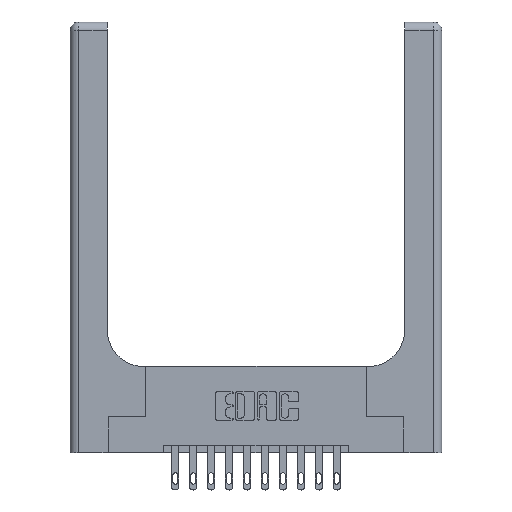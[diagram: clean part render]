
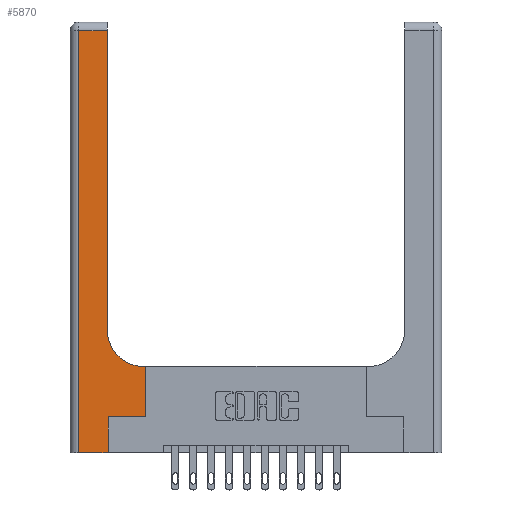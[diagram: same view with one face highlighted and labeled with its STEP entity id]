
A CAD part, top view. The second image highlights one B-rep face of the part: STEP entity #5870.
In plain terms, the highlighted planar face has unit normal (0, 0, 1).
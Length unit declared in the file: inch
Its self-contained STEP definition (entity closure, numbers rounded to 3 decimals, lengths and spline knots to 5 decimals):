
#575 = DIRECTION ( 'NONE',  ( 1., 0., 0. ) ) ;
#804 = LINE ( 'NONE', #5848, #12425 ) ;
#843 = VERTEX_POINT ( 'NONE', #5505 ) ;
#892 = LINE ( 'NONE', #11012, #16225 ) ;
#935 = CARTESIAN_POINT ( 'NONE',  ( 0.51, 0.85, 0.37 ) ) ;
#1201 = ORIENTED_EDGE ( 'NONE', *, *, #14154, .T. ) ;
#1214 = EDGE_CURVE ( 'NONE', #8845, #12951, #4245, .T. ) ;
#1396 = VECTOR ( 'NONE', #575, 39.37008 ) ;
#1635 = LINE ( 'NONE', #11578, #6724 ) ;
#1811 = CARTESIAN_POINT ( 'NONE',  ( 0.26, 2.94, 0.37 ) ) ;
#1819 = EDGE_CURVE ( 'NONE', #8567, #13595, #892, .T. ) ;
#1993 = VERTEX_POINT ( 'NONE', #1811 ) ;
#2097 = DIRECTION ( 'NONE',  ( 1., 0., 0. ) ) ;
#2362 = ORIENTED_EDGE ( 'NONE', *, *, #1819, .T. ) ;
#2417 = CARTESIAN_POINT ( 'NONE',  ( 0., 3., 0.37 ) ) ;
#3426 = EDGE_CURVE ( 'NONE', #12951, #843, #7021, .T. ) ;
#3713 = ORIENTED_EDGE ( 'NONE', *, *, #14754, .T. ) ;
#3787 = CIRCLE ( 'NONE', #14131, 0.25 ) ;
#4206 = CARTESIAN_POINT ( 'NONE',  ( 0.06, 2.94, 0.37 ) ) ;
#4245 = LINE ( 'NONE', #12049, #13888 ) ;
#4351 = VECTOR ( 'NONE', #10169, 39.37008 ) ;
#4692 = DIRECTION ( 'NONE',  ( 0., 1., 0. ) ) ;
#4849 = VECTOR ( 'NONE', #11426, 39.37008 ) ;
#5032 = CARTESIAN_POINT ( 'NONE',  ( 0.26, 3., 0.37 ) ) ;
#5188 = LINE ( 'NONE', #14057, #4351 ) ;
#5505 = CARTESIAN_POINT ( 'NONE',  ( 0.265, 0., 0.37 ) ) ;
#5636 = ORIENTED_EDGE ( 'NONE', *, *, #3426, .T. ) ;
#5846 = CARTESIAN_POINT ( 'NONE',  ( 0.51, 0.6, 0.37 ) ) ;
#5848 = CARTESIAN_POINT ( 'NONE',  ( 0.26, 0.6, 0.37 ) ) ;
#5870 = ADVANCED_FACE ( 'NONE', ( #5973 ), #8629, .F. ) ;
#5973 = FACE_OUTER_BOUND ( 'NONE', #10445, .T. ) ;
#6359 = LINE ( 'NONE', #5032, #4849 ) ;
#6724 = VECTOR ( 'NONE', #10414, 39.37008 ) ;
#7021 = LINE ( 'NONE', #11916, #1396 ) ;
#7136 = DIRECTION ( 'NONE',  ( 0., 0., -1. ) ) ;
#7688 = VERTEX_POINT ( 'NONE', #10016 ) ;
#7718 = DIRECTION ( 'NONE',  ( 1., 0., 0. ) ) ;
#7784 = CARTESIAN_POINT ( 'NONE',  ( 0.26, 0.85, 0.37 ) ) ;
#7898 = VERTEX_POINT ( 'NONE', #5846 ) ;
#8135 = CARTESIAN_POINT ( 'NONE',  ( 0.528, 0.25, 0.37 ) ) ;
#8567 = VERTEX_POINT ( 'NONE', #8135 ) ;
#8629 = PLANE ( 'NONE',  #15887 ) ;
#8845 = VERTEX_POINT ( 'NONE', #4206 ) ;
#8929 = ORIENTED_EDGE ( 'NONE', *, *, #9406, .T. ) ;
#8965 = ORIENTED_EDGE ( 'NONE', *, *, #1214, .T. ) ;
#9142 = EDGE_CURVE ( 'NONE', #13595, #7898, #804, .T. ) ;
#9253 = CARTESIAN_POINT ( 'NONE',  ( 0.06, 0., 0.37 ) ) ;
#9406 = EDGE_CURVE ( 'NONE', #1993, #8845, #5188, .T. ) ;
#9420 = EDGE_CURVE ( 'NONE', #843, #7688, #1635, .T. ) ;
#10016 = CARTESIAN_POINT ( 'NONE',  ( 0.265, 0.25, 0.37 ) ) ;
#10169 = DIRECTION ( 'NONE',  ( -1., 0., 0. ) ) ;
#10374 = DIRECTION ( 'NONE',  ( -1., 0., 0. ) ) ;
#10414 = DIRECTION ( 'NONE',  ( 0., 1., 0. ) ) ;
#10445 = EDGE_LOOP ( 'NONE', ( #1201, #8929, #8965, #5636, #11547, #3713, #2362, #16057, #12789 ) ) ;
#10460 = EDGE_CURVE ( 'NONE', #7898, #16153, #3787, .T. ) ;
#10917 = DIRECTION ( 'NONE',  ( -1., 0., 0. ) ) ;
#11012 = CARTESIAN_POINT ( 'NONE',  ( 0.528, 0.25, 0.37 ) ) ;
#11040 = DIRECTION ( 'NONE',  ( 0., 0., -1. ) ) ;
#11426 = DIRECTION ( 'NONE',  ( 0., 1., 0. ) ) ;
#11547 = ORIENTED_EDGE ( 'NONE', *, *, #9420, .T. ) ;
#11578 = CARTESIAN_POINT ( 'NONE',  ( 0.265, 0., 0.37 ) ) ;
#11614 = LINE ( 'NONE', #15094, #13357 ) ;
#11916 = CARTESIAN_POINT ( 'NONE',  ( 0., 0., 0.37 ) ) ;
#12049 = CARTESIAN_POINT ( 'NONE',  ( 0.06, 3., 0.37 ) ) ;
#12425 = VECTOR ( 'NONE', #10917, 39.37008 ) ;
#12789 = ORIENTED_EDGE ( 'NONE', *, *, #10460, .T. ) ;
#12951 = VERTEX_POINT ( 'NONE', #9253 ) ;
#13212 = DIRECTION ( 'NONE',  ( 0., -1., 0. ) ) ;
#13357 = VECTOR ( 'NONE', #7718, 39.37008 ) ;
#13595 = VERTEX_POINT ( 'NONE', #14830 ) ;
#13888 = VECTOR ( 'NONE', #13212, 39.37008 ) ;
#14057 = CARTESIAN_POINT ( 'NONE',  ( 0., 2.94, 0.37 ) ) ;
#14131 = AXIS2_PLACEMENT_3D ( 'NONE', #935, #7136, #2097 ) ;
#14154 = EDGE_CURVE ( 'NONE', #16153, #1993, #6359, .T. ) ;
#14754 = EDGE_CURVE ( 'NONE', #7688, #8567, #11614, .T. ) ;
#14830 = CARTESIAN_POINT ( 'NONE',  ( 0.528, 0.6, 0.37 ) ) ;
#15094 = CARTESIAN_POINT ( 'NONE',  ( 0.265, 0.25, 0.37 ) ) ;
#15887 = AXIS2_PLACEMENT_3D ( 'NONE', #2417, #11040, #10374 ) ;
#16057 = ORIENTED_EDGE ( 'NONE', *, *, #9142, .T. ) ;
#16153 = VERTEX_POINT ( 'NONE', #7784 ) ;
#16225 = VECTOR ( 'NONE', #4692, 39.37008 ) ;
